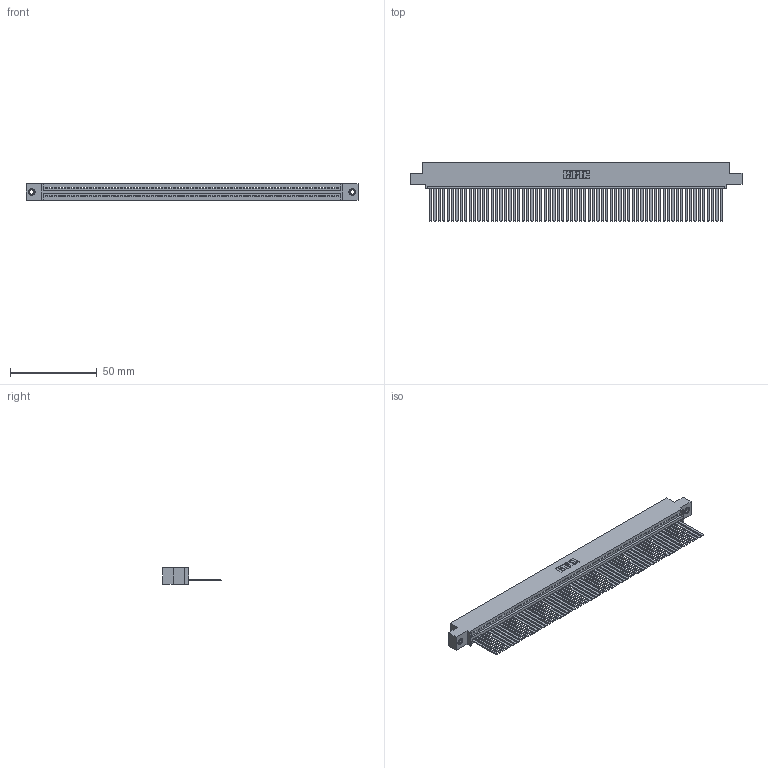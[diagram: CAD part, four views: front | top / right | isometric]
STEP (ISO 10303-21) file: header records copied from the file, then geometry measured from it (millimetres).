
FILE_DESCRIPTION (( 'STEP AP203' ), '1' );
FILE_NAME ('395-067-544-407.STEP', '2019-10-25T13:45:20', ( '' ), ( '' ), 'SwSTEP 2.0', 'SolidWorks 2016', '' );
FILE_SCHEMA (( 'CONFIG_CONTROL_DESIGN' ));
Length unit declared in the file: inch
Products named in the file (4): 345-250-001_345-250-005-103; 345 Part_0.110 Offset - 0.156 Dia-TI; 395-067-544-407; 345-292-001_345-293-144
Assembly tree (70 placements, depth 2):
  395-067-544-407
    345 Part_0.110 Offset - 0.156 Dia-TI
    345-292-001_345-293-144  x67
    345-250-001_345-250-005-103  x2
Bounding box: 191.39 x 33.96 x 9.4 mm (x, y, z)
Volume: 19072.2 mm3; surface area: 28128.9 mm2
Topology: 70 solids, 70 shells, 3674 faces, 11075 edges, 7286 vertices
Faces by surface type: plane 2528, cylinder 1130, cone 12, torus 4
Entity records: 48194 total; most frequent: CARTESIAN_POINT 8328, ORIENTED_EDGE 8322, DIRECTION 7261, EDGE_CURVE 4161, VECTOR 3745, LINE 3745, VERTEX_POINT 2768, AXIS2_PLACEMENT_3D 1758
